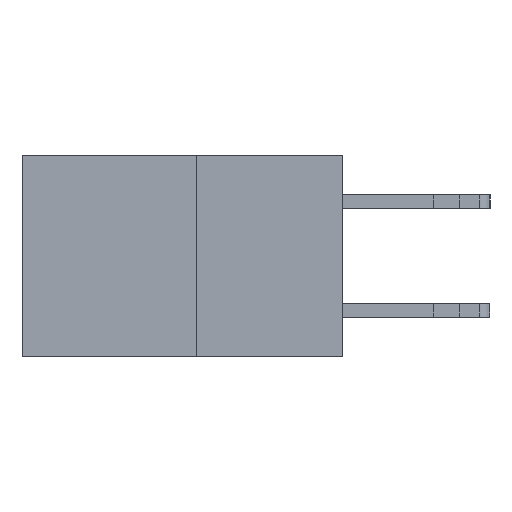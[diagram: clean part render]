
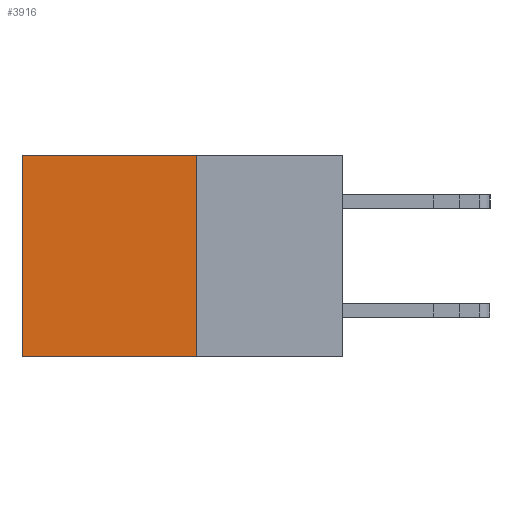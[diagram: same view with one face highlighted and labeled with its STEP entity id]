
A CAD part, left-side view. The second image highlights one B-rep face of the part: STEP entity #3916.
In plain terms, the highlighted planar face has unit normal (-1, 0, 0).
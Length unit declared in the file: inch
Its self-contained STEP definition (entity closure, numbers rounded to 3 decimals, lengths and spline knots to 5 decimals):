
#15 = DIRECTION ( 'NONE',  ( 0., 0., -1. ) ) ;
#362 = CARTESIAN_POINT ( 'NONE',  ( 0.277, 0.59, 0. ) ) ;
#618 = VECTOR ( 'NONE', #4372, 39.37008 ) ;
#681 = ORIENTED_EDGE ( 'NONE', *, *, #1006, .F. ) ;
#750 = CARTESIAN_POINT ( 'NONE',  ( 0.277, 0.27, 0. ) ) ;
#1006 = EDGE_CURVE ( 'NONE', #5615, #2353, #5099, .T. ) ;
#1065 = VERTEX_POINT ( 'NONE', #750 ) ;
#1066 = ORIENTED_EDGE ( 'NONE', *, *, #4071, .T. ) ;
#1430 = ORIENTED_EDGE ( 'NONE', *, *, #7534, .T. ) ;
#1984 = CARTESIAN_POINT ( 'NONE',  ( 0.277, 0.27, 0. ) ) ;
#2353 = VERTEX_POINT ( 'NONE', #5388 ) ;
#2743 = EDGE_CURVE ( 'NONE', #1065, #5615, #9150, .T. ) ;
#2901 = CARTESIAN_POINT ( 'NONE',  ( 0.277, 0.27, -0.37 ) ) ;
#2964 = PLANE ( 'NONE',  #7968 ) ;
#3776 = DIRECTION ( 'NONE',  ( 0., 1., 0. ) ) ;
#3916 = ADVANCED_FACE ( 'NONE', ( #11962 ), #2964, .F. ) ;
#4071 = EDGE_CURVE ( 'NONE', #1065, #5680, #5523, .T. ) ;
#4372 = DIRECTION ( 'NONE',  ( 0., 0., -1. ) ) ;
#5099 = LINE ( 'NONE', #10284, #9985 ) ;
#5106 = CARTESIAN_POINT ( 'NONE',  ( 0.277, 0.27, -0.37 ) ) ;
#5388 = CARTESIAN_POINT ( 'NONE',  ( 0.277, 0.59, -0.37 ) ) ;
#5523 = LINE ( 'NONE', #1984, #10389 ) ;
#5615 = VERTEX_POINT ( 'NONE', #5106 ) ;
#5680 = VERTEX_POINT ( 'NONE', #362 ) ;
#6440 = EDGE_LOOP ( 'NONE', ( #1430, #681, #11753, #1066 ) ) ;
#6559 = CARTESIAN_POINT ( 'NONE',  ( 0.277, 0.27, -0.37 ) ) ;
#7534 = EDGE_CURVE ( 'NONE', #5680, #2353, #11754, .T. ) ;
#7968 = AXIS2_PLACEMENT_3D ( 'NONE', #2901, #10456, #11008 ) ;
#8170 = CARTESIAN_POINT ( 'NONE',  ( 0.277, 0.59, -0.37 ) ) ;
#9063 = VECTOR ( 'NONE', #15, 39.37008 ) ;
#9150 = LINE ( 'NONE', #6559, #618 ) ;
#9743 = DIRECTION ( 'NONE',  ( 0., 1., 0. ) ) ;
#9985 = VECTOR ( 'NONE', #9743, 39.37008 ) ;
#10284 = CARTESIAN_POINT ( 'NONE',  ( 0.277, 0.27, -0.37 ) ) ;
#10389 = VECTOR ( 'NONE', #3776, 39.37008 ) ;
#10456 = DIRECTION ( 'NONE',  ( 1., 0., 0. ) ) ;
#11008 = DIRECTION ( 'NONE',  ( 0., 0., -1. ) ) ;
#11753 = ORIENTED_EDGE ( 'NONE', *, *, #2743, .F. ) ;
#11754 = LINE ( 'NONE', #8170, #9063 ) ;
#11962 = FACE_OUTER_BOUND ( 'NONE', #6440, .T. ) ;
